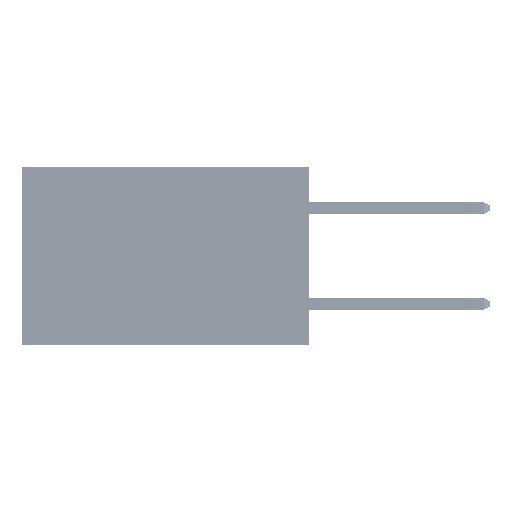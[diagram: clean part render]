
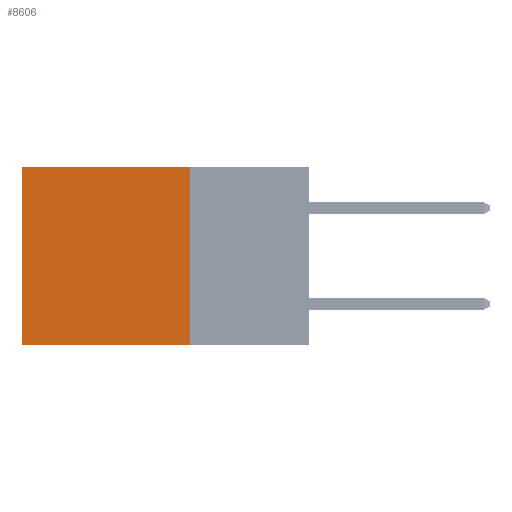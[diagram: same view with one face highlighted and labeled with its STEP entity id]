
A CAD part, left-side view. The second image highlights one B-rep face of the part: STEP entity #8606.
In plain terms, the highlighted planar face has unit normal (-1, 0, 0).
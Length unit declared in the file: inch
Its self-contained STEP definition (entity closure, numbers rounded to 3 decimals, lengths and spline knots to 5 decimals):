
#4113 = CARTESIAN_POINT ( 'NONE',  ( 0.2875, 0.25, 0. ) ) ;
#5792 = LINE ( 'NONE', #28128, #11492 ) ;
#5966 = VECTOR ( 'NONE', #26531, 39.37008 ) ;
#7444 = DIRECTION ( 'NONE',  ( 0., 0., -1. ) ) ;
#8345 = CARTESIAN_POINT ( 'NONE',  ( 0.2875, 0.6, -0.37 ) ) ;
#8523 = ORIENTED_EDGE ( 'NONE', *, *, #30292, .T. ) ;
#8606 = ADVANCED_FACE ( 'NONE', ( #32827 ), #17454, .F. ) ;
#11391 = CARTESIAN_POINT ( 'NONE',  ( 0.2875, 0.25, -0.37 ) ) ;
#11492 = VECTOR ( 'NONE', #17463, 39.37008 ) ;
#14215 = DIRECTION ( 'NONE',  ( 0., 0., -1. ) ) ;
#14899 = LINE ( 'NONE', #44927, #28179 ) ;
#17364 = VERTEX_POINT ( 'NONE', #8345 ) ;
#17454 = PLANE ( 'NONE',  #43710 ) ;
#17463 = DIRECTION ( 'NONE',  ( 0., 1., 0. ) ) ;
#18626 = ORIENTED_EDGE ( 'NONE', *, *, #48206, .T. ) ;
#24796 = CARTESIAN_POINT ( 'NONE',  ( 0.2875, 0.25, 0. ) ) ;
#25149 = DIRECTION ( 'NONE',  ( 1., 0., 0. ) ) ;
#25275 = LINE ( 'NONE', #24796, #45544 ) ;
#26252 = VERTEX_POINT ( 'NONE', #38254 ) ;
#26531 = DIRECTION ( 'NONE',  ( 0., 1., 0. ) ) ;
#28128 = CARTESIAN_POINT ( 'NONE',  ( 0.2875, 0.25, 0. ) ) ;
#28179 = VECTOR ( 'NONE', #7444, 39.37008 ) ;
#30292 = EDGE_CURVE ( 'NONE', #40296, #26252, #5792, .T. ) ;
#30610 = ORIENTED_EDGE ( 'NONE', *, *, #47496, .F. ) ;
#32262 = ORIENTED_EDGE ( 'NONE', *, *, #43003, .F. ) ;
#32827 = FACE_OUTER_BOUND ( 'NONE', #36974, .T. ) ;
#36974 = EDGE_LOOP ( 'NONE', ( #18626, #32262, #30610, #8523 ) ) ;
#37364 = CARTESIAN_POINT ( 'NONE',  ( 0.2875, 0.25, -0.37 ) ) ;
#37942 = LINE ( 'NONE', #11391, #5966 ) ;
#38254 = CARTESIAN_POINT ( 'NONE',  ( 0.2875, 0.6, 0. ) ) ;
#38897 = VERTEX_POINT ( 'NONE', #37364 ) ;
#39915 = DIRECTION ( 'NONE',  ( 0., 0., -1. ) ) ;
#40276 = CARTESIAN_POINT ( 'NONE',  ( 0.2875, 0.25, 0. ) ) ;
#40296 = VERTEX_POINT ( 'NONE', #4113 ) ;
#43003 = EDGE_CURVE ( 'NONE', #38897, #17364, #37942, .T. ) ;
#43710 = AXIS2_PLACEMENT_3D ( 'NONE', #40276, #25149, #14215 ) ;
#44927 = CARTESIAN_POINT ( 'NONE',  ( 0.2875, 0.6, 0. ) ) ;
#45544 = VECTOR ( 'NONE', #39915, 39.37008 ) ;
#47496 = EDGE_CURVE ( 'NONE', #40296, #38897, #25275, .T. ) ;
#48206 = EDGE_CURVE ( 'NONE', #26252, #17364, #14899, .T. ) ;
